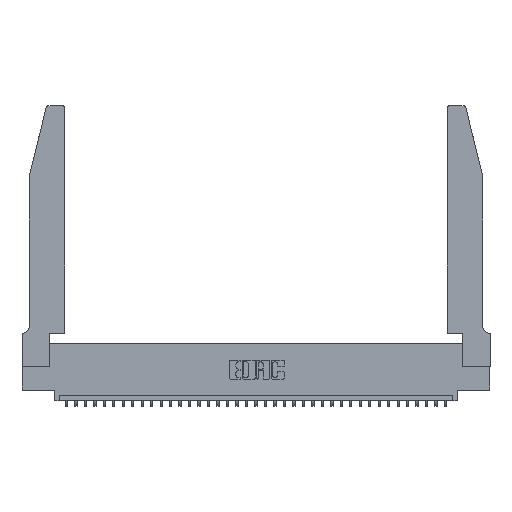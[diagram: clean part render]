
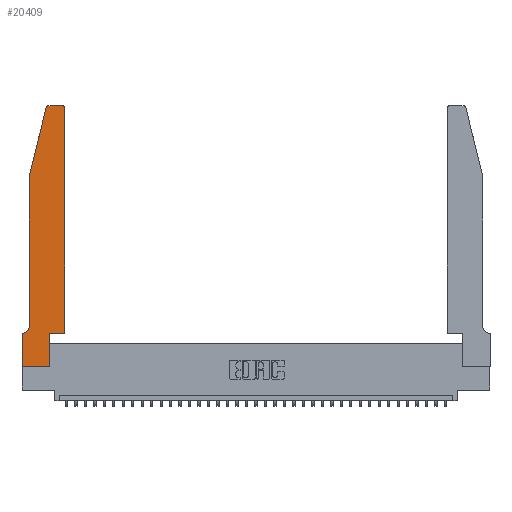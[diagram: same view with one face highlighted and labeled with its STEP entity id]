
A CAD part, top view. The second image highlights one B-rep face of the part: STEP entity #20409.
In plain terms, the highlighted planar face has unit normal (0, 0, 1).
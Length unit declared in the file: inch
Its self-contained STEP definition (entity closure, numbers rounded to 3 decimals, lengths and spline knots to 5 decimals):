
#32 = VERTEX_POINT ( 'NONE', #2033 ) ;
#63 = DIRECTION ( 'NONE',  ( -0.239, -0.971, 0. ) ) ;
#500 = VECTOR ( 'NONE', #63, 39.37008 ) ;
#1331 = ORIENTED_EDGE ( 'NONE', *, *, #5952, .T. ) ;
#1351 = DIRECTION ( 'NONE',  ( 0., 1., 0. ) ) ;
#2033 = CARTESIAN_POINT ( 'NONE',  ( 0.4505, 2.72, 0.37 ) ) ;
#2163 = VECTOR ( 'NONE', #1351, 39.37008 ) ;
#2418 = LINE ( 'NONE', #2524, #31072 ) ;
#2453 = LINE ( 'NONE', #19872, #31108 ) ;
#2524 = CARTESIAN_POINT ( 'NONE',  ( 0.4505, 0.35, 0.37 ) ) ;
#2729 = CARTESIAN_POINT ( 'NONE',  ( 0.2865, 0.35, 0.37 ) ) ;
#2773 = DIRECTION ( 'NONE',  ( 0., 1., 0. ) ) ;
#3276 = DIRECTION ( 'NONE',  ( 0., -1., 0. ) ) ;
#3305 = CARTESIAN_POINT ( 'NONE',  ( 0.2865, 0., 0.37 ) ) ;
#3380 = DIRECTION ( 'NONE',  ( 0., 0., -1. ) ) ;
#4487 = EDGE_CURVE ( 'NONE', #31320, #29148, #21849, .T. ) ;
#5315 = VECTOR ( 'NONE', #18665, 39.37008 ) ;
#5952 = EDGE_CURVE ( 'NONE', #11340, #31340, #14762, .T. ) ;
#6138 = VECTOR ( 'NONE', #8632, 39.37008 ) ;
#7168 = CARTESIAN_POINT ( 'NONE',  ( 0.2865, 0.35, 0.37 ) ) ;
#8104 = CIRCLE ( 'NONE', #24304, 0.07 ) ;
#8108 = CARTESIAN_POINT ( 'NONE',  ( 0.4505, 0.35, 0.37 ) ) ;
#8632 = DIRECTION ( 'NONE',  ( 1., 0., 0. ) ) ;
#8750 = CARTESIAN_POINT ( 'NONE',  ( 0.25487, 2.72718, 0.37 ) ) ;
#8872 = CARTESIAN_POINT ( 'NONE',  ( 0.0755, 0.42, 0.37 ) ) ;
#8874 = CARTESIAN_POINT ( 'NONE',  ( 0.284, 2.72, 0.37 ) ) ;
#8987 = DIRECTION ( 'NONE',  ( 0., 0., 1. ) ) ;
#9009 = EDGE_CURVE ( 'NONE', #30503, #32, #32210, .T. ) ;
#9802 = ORIENTED_EDGE ( 'NONE', *, *, #9009, .T. ) ;
#11340 = VERTEX_POINT ( 'NONE', #3305 ) ;
#11391 = EDGE_CURVE ( 'NONE', #32, #33605, #29827, .T. ) ;
#11397 = LINE ( 'NONE', #27846, #500 ) ;
#12864 = AXIS2_PLACEMENT_3D ( 'NONE', #25572, #8987, #28026 ) ;
#12965 = CARTESIAN_POINT ( 'NONE',  ( 0.4505, 0.35, 0.37 ) ) ;
#13250 = CARTESIAN_POINT ( 'NONE',  ( 0.2605, 2.75, 0.37 ) ) ;
#13451 = DIRECTION ( 'NONE',  ( 1., 0., 0. ) ) ;
#13609 = VECTOR ( 'NONE', #13802, 39.37008 ) ;
#13802 = DIRECTION ( 'NONE',  ( -1., 0., 0. ) ) ;
#14762 = LINE ( 'NONE', #7168, #2163 ) ;
#14845 = VERTEX_POINT ( 'NONE', #22189 ) ;
#15510 = ORIENTED_EDGE ( 'NONE', *, *, #23098, .T. ) ;
#15680 = ORIENTED_EDGE ( 'NONE', *, *, #18016, .T. ) ;
#17222 = ORIENTED_EDGE ( 'NONE', *, *, #35239, .T. ) ;
#17415 = FACE_OUTER_BOUND ( 'NONE', #34171, .T. ) ;
#17579 = EDGE_CURVE ( 'NONE', #29148, #35853, #2453, .T. ) ;
#18016 = EDGE_CURVE ( 'NONE', #31340, #30503, #2418, .T. ) ;
#18234 = LINE ( 'NONE', #28156, #34742 ) ;
#18651 = ORIENTED_EDGE ( 'NONE', *, *, #21993, .T. ) ;
#18665 = DIRECTION ( 'NONE',  ( -1., 0., 0. ) ) ;
#18929 = CARTESIAN_POINT ( 'NONE',  ( 0., 0.35, 0.37 ) ) ;
#19870 = DIRECTION ( 'NONE',  ( 1., 0., 0. ) ) ;
#19872 = CARTESIAN_POINT ( 'NONE',  ( 0., 0., 0.37 ) ) ;
#20003 = PLANE ( 'NONE',  #12864 ) ;
#20409 = ADVANCED_FACE ( 'NONE', ( #17415 ), #20003, .T. ) ;
#21075 = CARTESIAN_POINT ( 'NONE',  ( 0., 0., 0.37 ) ) ;
#21300 = ORIENTED_EDGE ( 'NONE', *, *, #11391, .T. ) ;
#21849 = LINE ( 'NONE', #25041, #13609 ) ;
#21993 = EDGE_CURVE ( 'NONE', #35853, #11340, #35666, .T. ) ;
#22189 = CARTESIAN_POINT ( 'NONE',  ( 0.0755, 2., 0.37 ) ) ;
#22434 = DIRECTION ( 'NONE',  ( 0., -1., 0. ) ) ;
#22544 = DIRECTION ( 'NONE',  ( 0., 0., 1. ) ) ;
#23098 = EDGE_CURVE ( 'NONE', #14845, #35567, #18234, .T. ) ;
#23196 = CARTESIAN_POINT ( 'NONE',  ( 0.284, 2.75, 0.37 ) ) ;
#24304 = AXIS2_PLACEMENT_3D ( 'NONE', #30804, #3380, #31055 ) ;
#24733 = ORIENTED_EDGE ( 'NONE', *, *, #30711, .T. ) ;
#25041 = CARTESIAN_POINT ( 'NONE',  ( 0.0755, 0.35, 0.37 ) ) ;
#25353 = EDGE_CURVE ( 'NONE', #35567, #31320, #8104, .T. ) ;
#25572 = CARTESIAN_POINT ( 'NONE',  ( 0., 0.35, 0.37 ) ) ;
#25723 = DIRECTION ( 'NONE',  ( 0., 0., 1. ) ) ;
#25811 = ORIENTED_EDGE ( 'NONE', *, *, #17579, .T. ) ;
#27196 = ORIENTED_EDGE ( 'NONE', *, *, #25353, .T. ) ;
#27243 = VERTEX_POINT ( 'NONE', #23196 ) ;
#27691 = CARTESIAN_POINT ( 'NONE',  ( 0.0055, 0.35, 0.37 ) ) ;
#27846 = CARTESIAN_POINT ( 'NONE',  ( 0.0755, 2., 0.37 ) ) ;
#28026 = DIRECTION ( 'NONE',  ( 1., 0., 0. ) ) ;
#28156 = CARTESIAN_POINT ( 'NONE',  ( 0.0755, 2., 0.37 ) ) ;
#28228 = AXIS2_PLACEMENT_3D ( 'NONE', #31096, #25723, #28418 ) ;
#28418 = DIRECTION ( 'NONE',  ( 1., 0., 0. ) ) ;
#28442 = CARTESIAN_POINT ( 'NONE',  ( 0.4205, 2.75, 0.37 ) ) ;
#29148 = VERTEX_POINT ( 'NONE', #18929 ) ;
#29190 = LINE ( 'NONE', #13250, #5315 ) ;
#29827 = CIRCLE ( 'NONE', #28228, 0.03 ) ;
#29915 = ORIENTED_EDGE ( 'NONE', *, *, #4487, .T. ) ;
#30048 = ORIENTED_EDGE ( 'NONE', *, *, #31871, .T. ) ;
#30115 = AXIS2_PLACEMENT_3D ( 'NONE', #8874, #22544, #19870 ) ;
#30503 = VERTEX_POINT ( 'NONE', #12965 ) ;
#30588 = CARTESIAN_POINT ( 'NONE',  ( 0., 0., 0.37 ) ) ;
#30711 = EDGE_CURVE ( 'NONE', #35452, #14845, #11397, .T. ) ;
#30804 = CARTESIAN_POINT ( 'NONE',  ( 0.0055, 0.42, 0.37 ) ) ;
#30905 = VECTOR ( 'NONE', #2773, 39.37008 ) ;
#31055 = DIRECTION ( 'NONE',  ( -1., 0., 0. ) ) ;
#31072 = VECTOR ( 'NONE', #13451, 39.37008 ) ;
#31096 = CARTESIAN_POINT ( 'NONE',  ( 0.4205, 2.72, 0.37 ) ) ;
#31108 = VECTOR ( 'NONE', #3276, 39.37008 ) ;
#31320 = VERTEX_POINT ( 'NONE', #27691 ) ;
#31340 = VERTEX_POINT ( 'NONE', #2729 ) ;
#31871 = EDGE_CURVE ( 'NONE', #33605, #27243, #29190, .T. ) ;
#32210 = LINE ( 'NONE', #8108, #30905 ) ;
#33605 = VERTEX_POINT ( 'NONE', #28442 ) ;
#34171 = EDGE_LOOP ( 'NONE', ( #30048, #17222, #24733, #15510, #27196, #29915, #25811, #18651, #1331, #15680, #9802, #21300 ) ) ;
#34742 = VECTOR ( 'NONE', #22434, 39.37008 ) ;
#35102 = CIRCLE ( 'NONE', #30115, 0.03 ) ;
#35239 = EDGE_CURVE ( 'NONE', #27243, #35452, #35102, .T. ) ;
#35452 = VERTEX_POINT ( 'NONE', #8750 ) ;
#35567 = VERTEX_POINT ( 'NONE', #8872 ) ;
#35666 = LINE ( 'NONE', #30588, #6138 ) ;
#35853 = VERTEX_POINT ( 'NONE', #21075 ) ;
